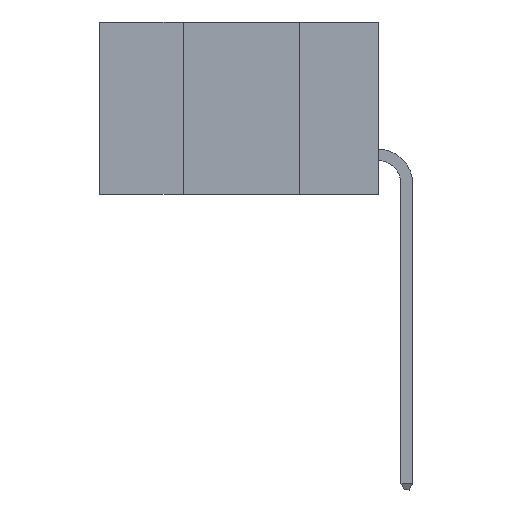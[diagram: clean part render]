
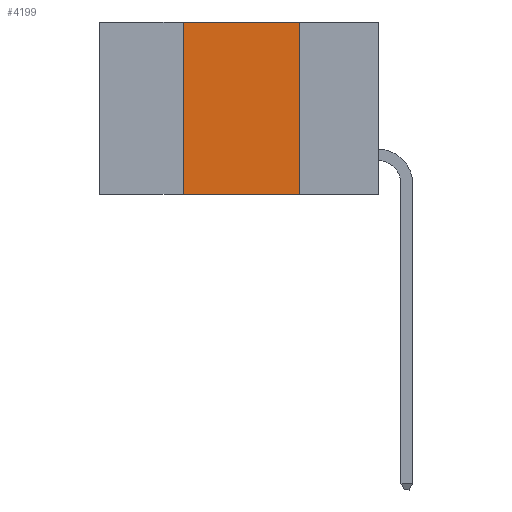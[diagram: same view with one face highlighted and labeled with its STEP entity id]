
A CAD part, left-side view. The second image highlights one B-rep face of the part: STEP entity #4199.
In plain terms, the highlighted planar face has unit normal (-1, 0, 0).
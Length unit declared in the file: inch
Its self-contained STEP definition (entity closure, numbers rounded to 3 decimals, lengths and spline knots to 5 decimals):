
#1681 = EDGE_CURVE ( 'NONE', #24155, #7455, #15868, .T. ) ;
#2849 = DIRECTION ( 'NONE',  ( 0., -1., 0. ) ) ;
#3388 = PLANE ( 'NONE',  #22275 ) ;
#3480 = CARTESIAN_POINT ( 'NONE',  ( 0., 0.6, 0. ) ) ;
#4199 = ADVANCED_FACE ( 'NONE', ( #21984 ), #3388, .F. ) ;
#4368 = DIRECTION ( 'NONE',  ( 0., 0., -1. ) ) ;
#5334 = CARTESIAN_POINT ( 'NONE',  ( 0., 0.42, -0.37 ) ) ;
#5446 = VECTOR ( 'NONE', #22542, 39.37008 ) ;
#7455 = VERTEX_POINT ( 'NONE', #24354 ) ;
#7688 = ORIENTED_EDGE ( 'NONE', *, *, #23135, .T. ) ;
#9745 = CARTESIAN_POINT ( 'NONE',  ( 0., 0.6, 0. ) ) ;
#10437 = VECTOR ( 'NONE', #2849, 39.37008 ) ;
#10698 = VECTOR ( 'NONE', #4368, 39.37008 ) ;
#13465 = LINE ( 'NONE', #27049, #5446 ) ;
#15484 = ORIENTED_EDGE ( 'NONE', *, *, #17371, .F. ) ;
#15868 = LINE ( 'NONE', #25356, #10698 ) ;
#16041 = ORIENTED_EDGE ( 'NONE', *, *, #29698, .F. ) ;
#16148 = CARTESIAN_POINT ( 'NONE',  ( 0., 0.42, 0. ) ) ;
#16697 = ORIENTED_EDGE ( 'NONE', *, *, #1681, .F. ) ;
#17371 = EDGE_CURVE ( 'NONE', #20627, #24155, #28711, .T. ) ;
#18306 = VERTEX_POINT ( 'NONE', #5334 ) ;
#19768 = DIRECTION ( 'NONE',  ( 1., 0., 0. ) ) ;
#20627 = VERTEX_POINT ( 'NONE', #16148 ) ;
#21487 = LINE ( 'NONE', #28734, #29172 ) ;
#21984 = FACE_OUTER_BOUND ( 'NONE', #29993, .T. ) ;
#22098 = DIRECTION ( 'NONE',  ( 0., 0., -1. ) ) ;
#22275 = AXIS2_PLACEMENT_3D ( 'NONE', #3480, #19768, #22098 ) ;
#22542 = DIRECTION ( 'NONE',  ( 0., 0., 1. ) ) ;
#23135 = EDGE_CURVE ( 'NONE', #18306, #7455, #21487, .T. ) ;
#23731 = DIRECTION ( 'NONE',  ( 0., -1., 0. ) ) ;
#23792 = CARTESIAN_POINT ( 'NONE',  ( 0., 0.17, 0. ) ) ;
#24155 = VERTEX_POINT ( 'NONE', #23792 ) ;
#24354 = CARTESIAN_POINT ( 'NONE',  ( 0., 0.17, -0.37 ) ) ;
#25356 = CARTESIAN_POINT ( 'NONE',  ( 0., 0.17, 0. ) ) ;
#27049 = CARTESIAN_POINT ( 'NONE',  ( 0., 0.42, 0. ) ) ;
#28711 = LINE ( 'NONE', #9745, #10437 ) ;
#28734 = CARTESIAN_POINT ( 'NONE',  ( 0., 0.6, -0.37 ) ) ;
#29172 = VECTOR ( 'NONE', #23731, 39.37008 ) ;
#29698 = EDGE_CURVE ( 'NONE', #18306, #20627, #13465, .T. ) ;
#29993 = EDGE_LOOP ( 'NONE', ( #16697, #15484, #16041, #7688 ) ) ;
